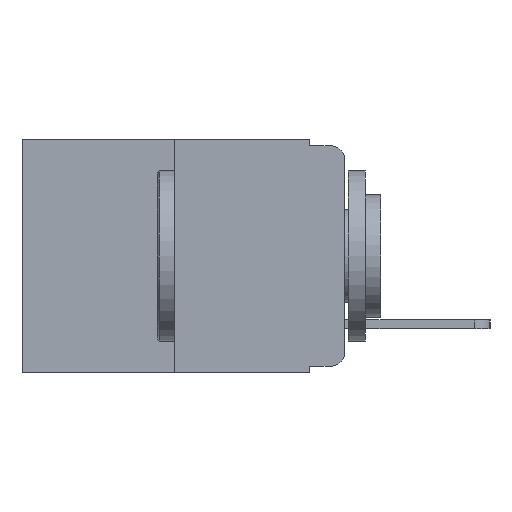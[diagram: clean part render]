
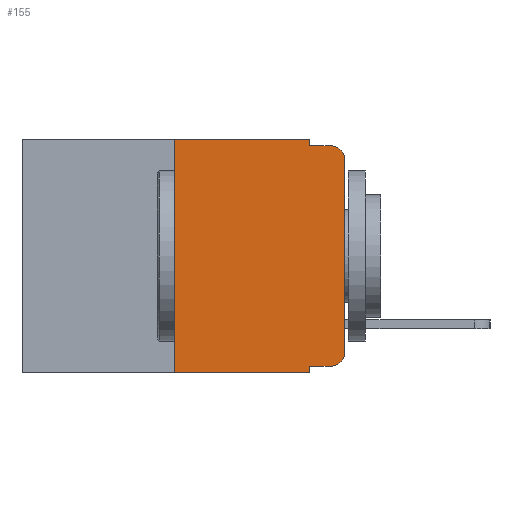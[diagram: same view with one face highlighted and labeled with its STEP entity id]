
A CAD part, left-side view. The second image highlights one B-rep face of the part: STEP entity #155.
In plain terms, the highlighted planar face has unit normal (-1, 0, 0).
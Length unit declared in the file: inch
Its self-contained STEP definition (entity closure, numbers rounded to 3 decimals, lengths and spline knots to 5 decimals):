
#2 = LINE ( 'NONE', #15305, #18141 ) ;
#20 = AXIS2_PLACEMENT_3D ( 'NONE', #2412, #2115, #2190 ) ;
#146 = EDGE_CURVE ( 'NONE', #14250, #9429, #3701, .T. ) ;
#155 = ADVANCED_FACE ( 'NONE', ( #14526 ), #2458, .F. ) ;
#265 = EDGE_CURVE ( 'NONE', #17272, #14250, #2, .T. ) ;
#793 = CARTESIAN_POINT ( 'NONE',  ( 0., 0.051, -0.333 ) ) ;
#1043 = CARTESIAN_POINT ( 'NONE',  ( 0., 0.25, -0.343 ) ) ;
#1407 = EDGE_CURVE ( 'NONE', #9429, #4903, #10843, .T. ) ;
#1742 = CIRCLE ( 'NONE', #5355, 0.02 ) ;
#2115 = DIRECTION ( 'NONE',  ( 1., 0., 0. ) ) ;
#2173 = CARTESIAN_POINT ( 'NONE',  ( 0., 0.051, -0.01 ) ) ;
#2190 = DIRECTION ( 'NONE',  ( 0., 0., -1. ) ) ;
#2412 = CARTESIAN_POINT ( 'NONE',  ( 0., 0.473, 0. ) ) ;
#2458 = PLANE ( 'NONE',  #20 ) ;
#2475 = EDGE_CURVE ( 'NONE', #4903, #6954, #3687, .T. ) ;
#2672 = DIRECTION ( 'NONE',  ( 0., 0., 1. ) ) ;
#2984 = LINE ( 'NONE', #4169, #10202 ) ;
#3190 = ORIENTED_EDGE ( 'NONE', *, *, #16980, .T. ) ;
#3258 = VECTOR ( 'NONE', #4901, 39.37008 ) ;
#3479 = EDGE_CURVE ( 'NONE', #3496, #6954, #1742, .T. ) ;
#3496 = VERTEX_POINT ( 'NONE', #16311 ) ;
#3687 = LINE ( 'NONE', #17920, #10015 ) ;
#3701 = LINE ( 'NONE', #5241, #3258 ) ;
#3842 = ORIENTED_EDGE ( 'NONE', *, *, #2475, .F. ) ;
#4053 = AXIS2_PLACEMENT_3D ( 'NONE', #15402, #7067, #16775 ) ;
#4169 = CARTESIAN_POINT ( 'NONE',  ( 0., 0.051, 0. ) ) ;
#4311 = ORIENTED_EDGE ( 'NONE', *, *, #1407, .F. ) ;
#4456 = EDGE_CURVE ( 'NONE', #10051, #3496, #10382, .T. ) ;
#4694 = VECTOR ( 'NONE', #15924, 39.37008 ) ;
#4759 = ORIENTED_EDGE ( 'NONE', *, *, #146, .F. ) ;
#4901 = DIRECTION ( 'NONE',  ( 0., -1., 0. ) ) ;
#4903 = VERTEX_POINT ( 'NONE', #2173 ) ;
#5241 = CARTESIAN_POINT ( 'NONE',  ( 0., 0.473, 0. ) ) ;
#5355 = AXIS2_PLACEMENT_3D ( 'NONE', #8040, #17654, #9475 ) ;
#5600 = CARTESIAN_POINT ( 'NONE',  ( 0., 0., 0. ) ) ;
#5636 = DIRECTION ( 'NONE',  ( 0., 0., -1. ) ) ;
#6036 = EDGE_CURVE ( 'NONE', #17272, #15431, #15887, .T. ) ;
#6474 = CARTESIAN_POINT ( 'NONE',  ( 0., 0., -0.313 ) ) ;
#6566 = VECTOR ( 'NONE', #2672, 39.37008 ) ;
#6686 = CARTESIAN_POINT ( 'NONE',  ( 0., 0.051, 0. ) ) ;
#6954 = VERTEX_POINT ( 'NONE', #16369 ) ;
#7067 = DIRECTION ( 'NONE',  ( -1., 0., 0. ) ) ;
#7489 = ORIENTED_EDGE ( 'NONE', *, *, #16069, .T. ) ;
#7818 = CARTESIAN_POINT ( 'NONE',  ( 0., 0.051, -0.333 ) ) ;
#8040 = CARTESIAN_POINT ( 'NONE',  ( 0., 0.02, -0.03 ) ) ;
#8613 = CARTESIAN_POINT ( 'NONE',  ( 0., 0.051, -0.343 ) ) ;
#8621 = ORIENTED_EDGE ( 'NONE', *, *, #265, .F. ) ;
#8838 = VERTEX_POINT ( 'NONE', #793 ) ;
#9008 = CARTESIAN_POINT ( 'NONE',  ( 0., 0.473, -0.343 ) ) ;
#9095 = VERTEX_POINT ( 'NONE', #10167 ) ;
#9255 = DIRECTION ( 'NONE',  ( 0., -1., 0. ) ) ;
#9429 = VERTEX_POINT ( 'NONE', #6686 ) ;
#9475 = DIRECTION ( 'NONE',  ( 0., 0., -1. ) ) ;
#9819 = DIRECTION ( 'NONE',  ( 0., -1., 0. ) ) ;
#10015 = VECTOR ( 'NONE', #9819, 39.37008 ) ;
#10051 = VERTEX_POINT ( 'NONE', #6474 ) ;
#10167 = CARTESIAN_POINT ( 'NONE',  ( 0., 0.02, -0.333 ) ) ;
#10202 = VECTOR ( 'NONE', #5636, 39.37008 ) ;
#10382 = LINE ( 'NONE', #5600, #6566 ) ;
#10411 = VECTOR ( 'NONE', #11846, 39.37008 ) ;
#10609 = ORIENTED_EDGE ( 'NONE', *, *, #4456, .T. ) ;
#10843 = LINE ( 'NONE', #11145, #10411 ) ;
#11145 = CARTESIAN_POINT ( 'NONE',  ( 0., 0.051, 0. ) ) ;
#11544 = LINE ( 'NONE', #7818, #14725 ) ;
#11846 = DIRECTION ( 'NONE',  ( 0., 0., -1. ) ) ;
#12337 = ORIENTED_EDGE ( 'NONE', *, *, #6036, .T. ) ;
#12940 = EDGE_LOOP ( 'NONE', ( #10609, #18260, #3842, #4311, #4759, #8621, #12337, #13193, #3190, #7489 ) ) ;
#13193 = ORIENTED_EDGE ( 'NONE', *, *, #17871, .F. ) ;
#14250 = VERTEX_POINT ( 'NONE', #14770 ) ;
#14341 = CIRCLE ( 'NONE', #4053, 0.02 ) ;
#14526 = FACE_OUTER_BOUND ( 'NONE', #12940, .T. ) ;
#14725 = VECTOR ( 'NONE', #9255, 39.37008 ) ;
#14770 = CARTESIAN_POINT ( 'NONE',  ( 0., 0.25, 0. ) ) ;
#15305 = CARTESIAN_POINT ( 'NONE',  ( 0., 0.25, 0. ) ) ;
#15402 = CARTESIAN_POINT ( 'NONE',  ( 0., 0.02, -0.313 ) ) ;
#15431 = VERTEX_POINT ( 'NONE', #8613 ) ;
#15708 = DIRECTION ( 'NONE',  ( 0., 0., 1. ) ) ;
#15887 = LINE ( 'NONE', #9008, #4694 ) ;
#15924 = DIRECTION ( 'NONE',  ( 0., -1., 0. ) ) ;
#16069 = EDGE_CURVE ( 'NONE', #9095, #10051, #14341, .T. ) ;
#16311 = CARTESIAN_POINT ( 'NONE',  ( 0., 0., -0.03 ) ) ;
#16369 = CARTESIAN_POINT ( 'NONE',  ( 0., 0.02, -0.01 ) ) ;
#16775 = DIRECTION ( 'NONE',  ( 0., 0., -1. ) ) ;
#16980 = EDGE_CURVE ( 'NONE', #8838, #9095, #11544, .T. ) ;
#17272 = VERTEX_POINT ( 'NONE', #1043 ) ;
#17654 = DIRECTION ( 'NONE',  ( -1., 0., 0. ) ) ;
#17871 = EDGE_CURVE ( 'NONE', #8838, #15431, #2984, .T. ) ;
#17920 = CARTESIAN_POINT ( 'NONE',  ( 0., 0.051, -0.01 ) ) ;
#18141 = VECTOR ( 'NONE', #15708, 39.37008 ) ;
#18260 = ORIENTED_EDGE ( 'NONE', *, *, #3479, .T. ) ;
